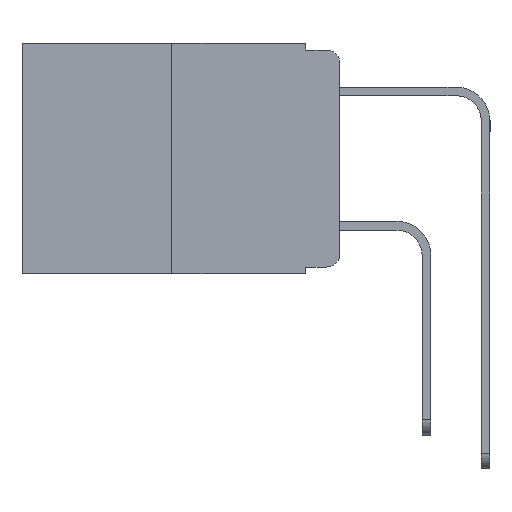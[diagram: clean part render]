
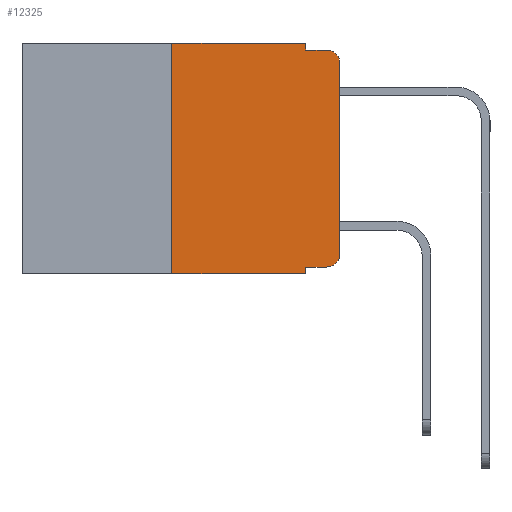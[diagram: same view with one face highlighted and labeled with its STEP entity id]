
A CAD part, left-side view. The second image highlights one B-rep face of the part: STEP entity #12325.
In plain terms, the highlighted planar face has unit normal (-1, 0, 0).
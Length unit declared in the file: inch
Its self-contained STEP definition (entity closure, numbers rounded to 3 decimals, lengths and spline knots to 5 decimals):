
#44 = DIRECTION ( 'NONE',  ( 0., 0., -1. ) ) ;
#498 = CARTESIAN_POINT ( 'NONE',  ( 0., 0., -0.313 ) ) ;
#522 = CARTESIAN_POINT ( 'NONE',  ( 0., 0.25, -0.343 ) ) ;
#1077 = EDGE_CURVE ( 'NONE', #16469, #1393, #12425, .T. ) ;
#1148 = DIRECTION ( 'NONE',  ( 0., -1., 0. ) ) ;
#1250 = DIRECTION ( 'NONE',  ( -1., 0., 0. ) ) ;
#1361 = CARTESIAN_POINT ( 'NONE',  ( 0., 0.02, -0.333 ) ) ;
#1393 = VERTEX_POINT ( 'NONE', #15070 ) ;
#1503 = VECTOR ( 'NONE', #11784, 39.37008 ) ;
#1551 = VECTOR ( 'NONE', #1148, 39.37008 ) ;
#1780 = DIRECTION ( 'NONE',  ( -1., 0., 0. ) ) ;
#1875 = DIRECTION ( 'NONE',  ( 0., 0., 1. ) ) ;
#1915 = CARTESIAN_POINT ( 'NONE',  ( 0., 0., 0. ) ) ;
#1996 = VERTEX_POINT ( 'NONE', #2589 ) ;
#2104 = EDGE_CURVE ( 'NONE', #9428, #1393, #6285, .T. ) ;
#2211 = CARTESIAN_POINT ( 'NONE',  ( 0., 0.051, -0.01 ) ) ;
#2235 = VECTOR ( 'NONE', #6055, 39.37008 ) ;
#2258 = CARTESIAN_POINT ( 'NONE',  ( 0., 0.051, 0. ) ) ;
#2276 = DIRECTION ( 'NONE',  ( 0., 0., -1. ) ) ;
#2332 = CARTESIAN_POINT ( 'NONE',  ( 0., 0.051, -0.333 ) ) ;
#2377 = LINE ( 'NONE', #16144, #15767 ) ;
#2589 = CARTESIAN_POINT ( 'NONE',  ( 0., 0.051, -0.343 ) ) ;
#3075 = PLANE ( 'NONE',  #4140 ) ;
#3088 = EDGE_CURVE ( 'NONE', #9347, #9428, #7081, .T. ) ;
#3254 = VERTEX_POINT ( 'NONE', #9679 ) ;
#4070 = ORIENTED_EDGE ( 'NONE', *, *, #3088, .T. ) ;
#4140 = AXIS2_PLACEMENT_3D ( 'NONE', #11164, #8593, #44 ) ;
#4471 = EDGE_CURVE ( 'NONE', #14347, #14511, #16365, .T. ) ;
#5096 = VERTEX_POINT ( 'NONE', #1361 ) ;
#5660 = ORIENTED_EDGE ( 'NONE', *, *, #16297, .F. ) ;
#5830 = ORIENTED_EDGE ( 'NONE', *, *, #4471, .F. ) ;
#5847 = ORIENTED_EDGE ( 'NONE', *, *, #2104, .T. ) ;
#5855 = LINE ( 'NONE', #10806, #1551 ) ;
#5903 = ORIENTED_EDGE ( 'NONE', *, *, #10586, .T. ) ;
#5970 = CARTESIAN_POINT ( 'NONE',  ( 0., 0.051, 0. ) ) ;
#6044 = ORIENTED_EDGE ( 'NONE', *, *, #13204, .T. ) ;
#6055 = DIRECTION ( 'NONE',  ( 0., -1., 0. ) ) ;
#6072 = ORIENTED_EDGE ( 'NONE', *, *, #14776, .F. ) ;
#6241 = ORIENTED_EDGE ( 'NONE', *, *, #12368, .T. ) ;
#6285 = CIRCLE ( 'NONE', #16426, 0.02 ) ;
#6528 = LINE ( 'NONE', #2258, #13374 ) ;
#6852 = CARTESIAN_POINT ( 'NONE',  ( 0., 0.051, 0. ) ) ;
#7081 = LINE ( 'NONE', #1915, #10562 ) ;
#7315 = DIRECTION ( 'NONE',  ( 0., 0., -1. ) ) ;
#7473 = VECTOR ( 'NONE', #7315, 39.37008 ) ;
#7741 = CARTESIAN_POINT ( 'NONE',  ( 0., 0., -0.03 ) ) ;
#7894 = ORIENTED_EDGE ( 'NONE', *, *, #7998, .F. ) ;
#7914 = ORIENTED_EDGE ( 'NONE', *, *, #1077, .F. ) ;
#7946 = VERTEX_POINT ( 'NONE', #522 ) ;
#7998 = EDGE_CURVE ( 'NONE', #14511, #16469, #6528, .T. ) ;
#8593 = DIRECTION ( 'NONE',  ( 1., 0., 0. ) ) ;
#8613 = CARTESIAN_POINT ( 'NONE',  ( 0., 0.473, 0. ) ) ;
#8659 = AXIS2_PLACEMENT_3D ( 'NONE', #10020, #1780, #11338 ) ;
#9177 = FACE_OUTER_BOUND ( 'NONE', #11245, .T. ) ;
#9347 = VERTEX_POINT ( 'NONE', #498 ) ;
#9424 = VECTOR ( 'NONE', #16451, 39.37008 ) ;
#9428 = VERTEX_POINT ( 'NONE', #7741 ) ;
#9679 = CARTESIAN_POINT ( 'NONE',  ( 0., 0.051, -0.333 ) ) ;
#10020 = CARTESIAN_POINT ( 'NONE',  ( 0., 0.02, -0.313 ) ) ;
#10562 = VECTOR ( 'NONE', #1875, 39.37008 ) ;
#10586 = EDGE_CURVE ( 'NONE', #7946, #1996, #5855, .T. ) ;
#10806 = CARTESIAN_POINT ( 'NONE',  ( 0., 0.473, -0.343 ) ) ;
#11164 = CARTESIAN_POINT ( 'NONE',  ( 0., 0.473, 0. ) ) ;
#11245 = EDGE_LOOP ( 'NONE', ( #4070, #5847, #7914, #7894, #5830, #5660, #5903, #6072, #6044, #6241 ) ) ;
#11338 = DIRECTION ( 'NONE',  ( 0., 0., -1. ) ) ;
#11719 = DIRECTION ( 'NONE',  ( 0., 0., -1. ) ) ;
#11784 = DIRECTION ( 'NONE',  ( 0., -1., 0. ) ) ;
#11787 = CIRCLE ( 'NONE', #8659, 0.02 ) ;
#12325 = ADVANCED_FACE ( 'NONE', ( #9177 ), #3075, .F. ) ;
#12368 = EDGE_CURVE ( 'NONE', #5096, #9347, #11787, .T. ) ;
#12425 = LINE ( 'NONE', #16502, #9424 ) ;
#13204 = EDGE_CURVE ( 'NONE', #3254, #5096, #15114, .T. ) ;
#13374 = VECTOR ( 'NONE', #11719, 39.37008 ) ;
#13756 = CARTESIAN_POINT ( 'NONE',  ( 0., 0.02, -0.03 ) ) ;
#14347 = VERTEX_POINT ( 'NONE', #15343 ) ;
#14511 = VERTEX_POINT ( 'NONE', #6852 ) ;
#14776 = EDGE_CURVE ( 'NONE', #3254, #1996, #16858, .T. ) ;
#15044 = DIRECTION ( 'NONE',  ( 0., 0., 1. ) ) ;
#15070 = CARTESIAN_POINT ( 'NONE',  ( 0., 0.02, -0.01 ) ) ;
#15114 = LINE ( 'NONE', #2332, #1503 ) ;
#15343 = CARTESIAN_POINT ( 'NONE',  ( 0., 0.25, 0. ) ) ;
#15767 = VECTOR ( 'NONE', #15044, 39.37008 ) ;
#16144 = CARTESIAN_POINT ( 'NONE',  ( 0., 0.25, 0. ) ) ;
#16297 = EDGE_CURVE ( 'NONE', #7946, #14347, #2377, .T. ) ;
#16365 = LINE ( 'NONE', #8613, #2235 ) ;
#16426 = AXIS2_PLACEMENT_3D ( 'NONE', #13756, #1250, #2276 ) ;
#16451 = DIRECTION ( 'NONE',  ( 0., -1., 0. ) ) ;
#16469 = VERTEX_POINT ( 'NONE', #2211 ) ;
#16502 = CARTESIAN_POINT ( 'NONE',  ( 0., 0.051, -0.01 ) ) ;
#16858 = LINE ( 'NONE', #5970, #7473 ) ;
